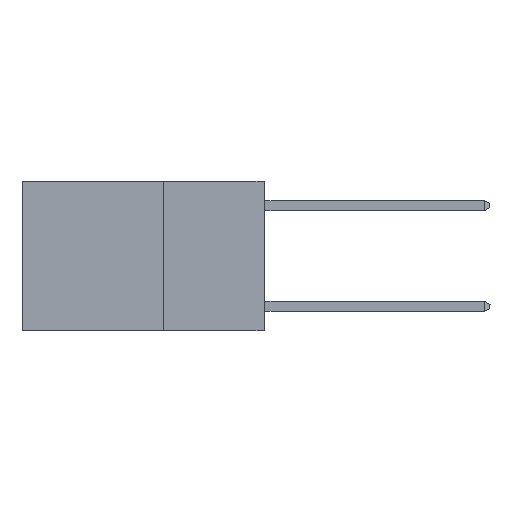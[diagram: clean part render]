
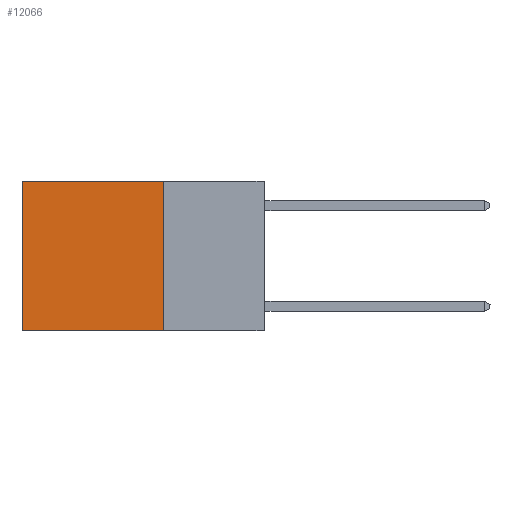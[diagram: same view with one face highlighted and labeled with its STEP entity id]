
A CAD part, left-side view. The second image highlights one B-rep face of the part: STEP entity #12066.
In plain terms, the highlighted planar face has unit normal (-1, 0, 0).
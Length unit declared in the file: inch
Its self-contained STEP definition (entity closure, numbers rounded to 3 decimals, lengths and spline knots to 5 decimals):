
#1 = CARTESIAN_POINT ( 'NONE',  ( 0.2625, 0.25, 0. ) ) ;
#817 = CARTESIAN_POINT ( 'NONE',  ( 0.2625, 0.25, 0. ) ) ;
#965 = CARTESIAN_POINT ( 'NONE',  ( 0.2625, 0.6, -0.37 ) ) ;
#1825 = ORIENTED_EDGE ( 'NONE', *, *, #13092, .T. ) ;
#2098 = ORIENTED_EDGE ( 'NONE', *, *, #16356, .T. ) ;
#2798 = CARTESIAN_POINT ( 'NONE',  ( 0.2625, 0.25, 0. ) ) ;
#3435 = PLANE ( 'NONE',  #16507 ) ;
#4385 = LINE ( 'NONE', #8987, #11445 ) ;
#5014 = FACE_OUTER_BOUND ( 'NONE', #10557, .T. ) ;
#5607 = VECTOR ( 'NONE', #10251, 39.37008 ) ;
#7698 = VERTEX_POINT ( 'NONE', #965 ) ;
#7755 = DIRECTION ( 'NONE',  ( 0., 1., 0. ) ) ;
#8063 = CARTESIAN_POINT ( 'NONE',  ( 0.2625, 0.6, 0. ) ) ;
#8228 = CARTESIAN_POINT ( 'NONE',  ( 0.2625, 0.25, -0.37 ) ) ;
#8615 = CARTESIAN_POINT ( 'NONE',  ( 0.2625, 0.6, 0. ) ) ;
#8898 = VERTEX_POINT ( 'NONE', #8063 ) ;
#8987 = CARTESIAN_POINT ( 'NONE',  ( 0.2625, 0.25, -0.37 ) ) ;
#10251 = DIRECTION ( 'NONE',  ( 0., 0., -1. ) ) ;
#10320 = LINE ( 'NONE', #2798, #12109 ) ;
#10557 = EDGE_LOOP ( 'NONE', ( #1825, #11819, #15340, #2098 ) ) ;
#10729 = EDGE_CURVE ( 'NONE', #14503, #12084, #10320, .T. ) ;
#11445 = VECTOR ( 'NONE', #7755, 39.37008 ) ;
#11670 = LINE ( 'NONE', #8615, #5607 ) ;
#11819 = ORIENTED_EDGE ( 'NONE', *, *, #13834, .F. ) ;
#12066 = ADVANCED_FACE ( 'NONE', ( #5014 ), #3435, .F. ) ;
#12084 = VERTEX_POINT ( 'NONE', #8228 ) ;
#12109 = VECTOR ( 'NONE', #13154, 39.37008 ) ;
#12345 = VECTOR ( 'NONE', #13669, 39.37008 ) ;
#12491 = DIRECTION ( 'NONE',  ( 1., 0., 0. ) ) ;
#13092 = EDGE_CURVE ( 'NONE', #8898, #7698, #11670, .T. ) ;
#13154 = DIRECTION ( 'NONE',  ( 0., 0., -1. ) ) ;
#13669 = DIRECTION ( 'NONE',  ( 0., 1., 0. ) ) ;
#13834 = EDGE_CURVE ( 'NONE', #12084, #7698, #4385, .T. ) ;
#14503 = VERTEX_POINT ( 'NONE', #1 ) ;
#14641 = DIRECTION ( 'NONE',  ( 0., 0., -1. ) ) ;
#15340 = ORIENTED_EDGE ( 'NONE', *, *, #10729, .F. ) ;
#15752 = LINE ( 'NONE', #817, #12345 ) ;
#15900 = CARTESIAN_POINT ( 'NONE',  ( 0.2625, 0.25, 0. ) ) ;
#16356 = EDGE_CURVE ( 'NONE', #14503, #8898, #15752, .T. ) ;
#16507 = AXIS2_PLACEMENT_3D ( 'NONE', #15900, #12491, #14641 ) ;
